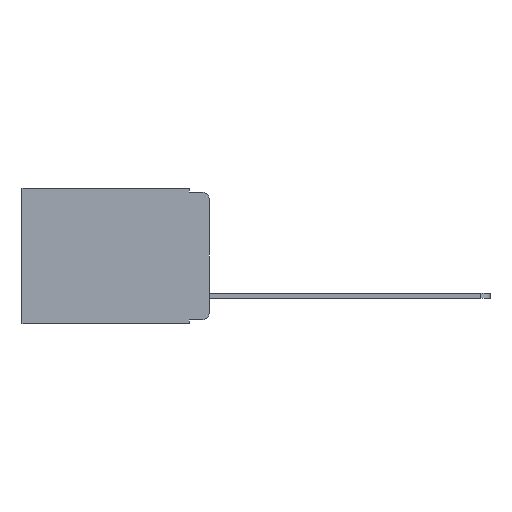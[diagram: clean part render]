
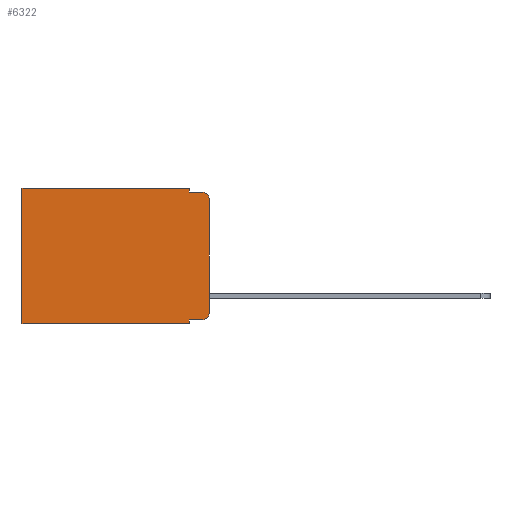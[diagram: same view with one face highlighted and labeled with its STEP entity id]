
A CAD part, left-side view. The second image highlights one B-rep face of the part: STEP entity #6322.
In plain terms, the highlighted planar face has unit normal (-1, 0, 0).
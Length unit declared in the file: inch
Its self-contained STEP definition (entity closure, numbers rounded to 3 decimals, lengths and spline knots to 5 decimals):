
#28 = VECTOR ( 'NONE', #4214, 39.37008 ) ;
#55 = DIRECTION ( 'NONE',  ( -1., 0., 0. ) ) ;
#217 = VERTEX_POINT ( 'NONE', #5507 ) ;
#239 = AXIS2_PLACEMENT_3D ( 'NONE', #11953, #55, #3247 ) ;
#490 = CARTESIAN_POINT ( 'NONE',  ( 0.298, 0., -0.313 ) ) ;
#651 = EDGE_CURVE ( 'NONE', #4021, #2637, #9980, .T. ) ;
#660 = EDGE_CURVE ( 'NONE', #4021, #2233, #4588, .T. ) ;
#702 = CIRCLE ( 'NONE', #239, 0.02 ) ;
#734 = EDGE_CURVE ( 'NONE', #2637, #12591, #702, .T. ) ;
#780 = EDGE_CURVE ( 'NONE', #7946, #217, #8256, .T. ) ;
#784 = EDGE_CURVE ( 'NONE', #12602, #9895, #12481, .T. ) ;
#785 = EDGE_CURVE ( 'NONE', #9895, #4561, #10389, .T. ) ;
#799 = CARTESIAN_POINT ( 'NONE',  ( 0.298, 0.051, -0.01 ) ) ;
#999 = EDGE_CURVE ( 'NONE', #8414, #4561, #11496, .T. ) ;
#1335 = CARTESIAN_POINT ( 'NONE',  ( 0.298, 0., -0.343 ) ) ;
#1798 = VECTOR ( 'NONE', #9819, 39.37008 ) ;
#1816 = VECTOR ( 'NONE', #5341, 39.37008 ) ;
#1830 = DIRECTION ( 'NONE',  ( 0., 0., -1. ) ) ;
#1867 = ORIENTED_EDGE ( 'NONE', *, *, #4982, .F. ) ;
#2233 = VERTEX_POINT ( 'NONE', #10873 ) ;
#2288 = AXIS2_PLACEMENT_3D ( 'NONE', #11513, #10274, #2566 ) ;
#2355 = DIRECTION ( 'NONE',  ( 1., 0., 0. ) ) ;
#2367 = CARTESIAN_POINT ( 'NONE',  ( 0.298, 0.02, -0.333 ) ) ;
#2555 = ORIENTED_EDGE ( 'NONE', *, *, #11789, .F. ) ;
#2564 = DIRECTION ( 'NONE',  ( 0., 0., -1. ) ) ;
#2566 = DIRECTION ( 'NONE',  ( 0., 0., -1. ) ) ;
#2637 = VERTEX_POINT ( 'NONE', #2367 ) ;
#2683 = PLANE ( 'NONE',  #9055 ) ;
#2851 = ORIENTED_EDGE ( 'NONE', *, *, #660, .F. ) ;
#3217 = CARTESIAN_POINT ( 'NONE',  ( 0.298, 0.051, -0.01 ) ) ;
#3247 = DIRECTION ( 'NONE',  ( 0., 0., -1. ) ) ;
#3260 = CARTESIAN_POINT ( 'NONE',  ( 0.298, 0., 0. ) ) ;
#3270 = EDGE_LOOP ( 'NONE', ( #1867, #10993, #4634, #10026, #4942, #12393, #2555, #2851, #5570, #5879 ) ) ;
#3393 = VECTOR ( 'NONE', #8403, 39.37008 ) ;
#4021 = VERTEX_POINT ( 'NONE', #11868 ) ;
#4214 = DIRECTION ( 'NONE',  ( 0., 0., -1. ) ) ;
#4561 = VERTEX_POINT ( 'NONE', #4859 ) ;
#4588 = LINE ( 'NONE', #5645, #1816 ) ;
#4634 = ORIENTED_EDGE ( 'NONE', *, *, #785, .F. ) ;
#4792 = CARTESIAN_POINT ( 'NONE',  ( 0.298, 0.051, 0. ) ) ;
#4859 = CARTESIAN_POINT ( 'NONE',  ( 0.298, 0.02, -0.01 ) ) ;
#4942 = ORIENTED_EDGE ( 'NONE', *, *, #9787, .T. ) ;
#4982 = EDGE_CURVE ( 'NONE', #8414, #12591, #10722, .T. ) ;
#5020 = CARTESIAN_POINT ( 'NONE',  ( 0.298, 0.051, -0.333 ) ) ;
#5341 = DIRECTION ( 'NONE',  ( 0., 0., -1. ) ) ;
#5366 = VECTOR ( 'NONE', #8532, 39.37008 ) ;
#5507 = CARTESIAN_POINT ( 'NONE',  ( 0.298, 0.473, -0.343 ) ) ;
#5570 = ORIENTED_EDGE ( 'NONE', *, *, #651, .T. ) ;
#5589 = FACE_OUTER_BOUND ( 'NONE', #3270, .T. ) ;
#5645 = CARTESIAN_POINT ( 'NONE',  ( 0.298, 0.051, 0. ) ) ;
#5764 = LINE ( 'NONE', #1335, #3393 ) ;
#5783 = CARTESIAN_POINT ( 'NONE',  ( 0.298, 0., 0. ) ) ;
#5879 = ORIENTED_EDGE ( 'NONE', *, *, #734, .T. ) ;
#6020 = CARTESIAN_POINT ( 'NONE',  ( 0.298, 0., 0. ) ) ;
#6322 = ADVANCED_FACE ( 'NONE', ( #5589 ), #2683, .F. ) ;
#7177 = VECTOR ( 'NONE', #8696, 39.37008 ) ;
#7626 = VECTOR ( 'NONE', #8849, 39.37008 ) ;
#7794 = CARTESIAN_POINT ( 'NONE',  ( 0.298, 0.051, 0. ) ) ;
#7942 = VECTOR ( 'NONE', #1830, 39.37008 ) ;
#7946 = VERTEX_POINT ( 'NONE', #8574 ) ;
#8256 = LINE ( 'NONE', #11472, #7942 ) ;
#8403 = DIRECTION ( 'NONE',  ( 0., 1., 0. ) ) ;
#8414 = VERTEX_POINT ( 'NONE', #11281 ) ;
#8532 = DIRECTION ( 'NONE',  ( 0., 0., -1. ) ) ;
#8574 = CARTESIAN_POINT ( 'NONE',  ( 0.298, 0.473, 0. ) ) ;
#8696 = DIRECTION ( 'NONE',  ( 0., -1., 0. ) ) ;
#8849 = DIRECTION ( 'NONE',  ( 0., -1., 0. ) ) ;
#9055 = AXIS2_PLACEMENT_3D ( 'NONE', #3260, #2355, #2564 ) ;
#9787 = EDGE_CURVE ( 'NONE', #12602, #7946, #12070, .T. ) ;
#9819 = DIRECTION ( 'NONE',  ( 0., 1., 0. ) ) ;
#9895 = VERTEX_POINT ( 'NONE', #3217 ) ;
#9980 = LINE ( 'NONE', #5020, #7177 ) ;
#10026 = ORIENTED_EDGE ( 'NONE', *, *, #784, .F. ) ;
#10274 = DIRECTION ( 'NONE',  ( -1., 0., 0. ) ) ;
#10389 = LINE ( 'NONE', #799, #7626 ) ;
#10722 = LINE ( 'NONE', #5783, #28 ) ;
#10873 = CARTESIAN_POINT ( 'NONE',  ( 0.298, 0.051, -0.343 ) ) ;
#10993 = ORIENTED_EDGE ( 'NONE', *, *, #999, .T. ) ;
#11281 = CARTESIAN_POINT ( 'NONE',  ( 0.298, 0., -0.03 ) ) ;
#11472 = CARTESIAN_POINT ( 'NONE',  ( 0.298, 0.473, 0. ) ) ;
#11496 = CIRCLE ( 'NONE', #2288, 0.02 ) ;
#11513 = CARTESIAN_POINT ( 'NONE',  ( 0.298, 0.02, -0.03 ) ) ;
#11789 = EDGE_CURVE ( 'NONE', #2233, #217, #5764, .T. ) ;
#11868 = CARTESIAN_POINT ( 'NONE',  ( 0.298, 0.051, -0.333 ) ) ;
#11953 = CARTESIAN_POINT ( 'NONE',  ( 0.298, 0.02, -0.313 ) ) ;
#12070 = LINE ( 'NONE', #6020, #1798 ) ;
#12393 = ORIENTED_EDGE ( 'NONE', *, *, #780, .T. ) ;
#12481 = LINE ( 'NONE', #7794, #5366 ) ;
#12591 = VERTEX_POINT ( 'NONE', #490 ) ;
#12602 = VERTEX_POINT ( 'NONE', #4792 ) ;
